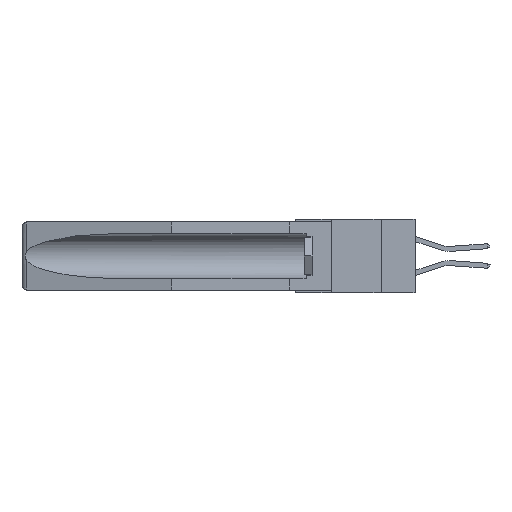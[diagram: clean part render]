
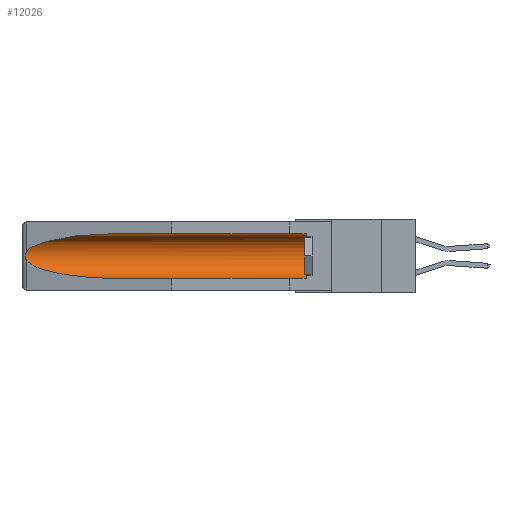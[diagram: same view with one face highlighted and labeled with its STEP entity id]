
A CAD part, left-side view. The second image highlights one B-rep face of the part: STEP entity #12026.
In plain terms, the highlighted cylindrical face has radius 2.857 mm (diameter 5.715 mm), a partial arc.
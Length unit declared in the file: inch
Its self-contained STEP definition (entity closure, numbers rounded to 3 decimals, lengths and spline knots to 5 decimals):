
#19 = CARTESIAN_POINT ( 'NONE',  ( 0.155, -0.30754, -0.059 ) ) ;
#221 = DIRECTION ( 'NONE',  ( 0., 1., 0. ) ) ;
#250 = VERTEX_POINT ( 'NONE', #28380 ) ;
#555 = EDGE_CURVE ( 'NONE', #11129, #9477, #27718, .T. ) ;
#1300 = ORIENTED_EDGE ( 'NONE', *, *, #555, .T. ) ;
#1392 = CARTESIAN_POINT ( 'NONE',  ( 0.25451, 1.48313, -0.09465 ) ) ;
#1483 = CARTESIAN_POINT ( 'NONE',  ( 0.21114, 1.30732, -0.059 ) ) ;
#3285 = DIRECTION ( 'NONE',  ( 0., 1., 0. ) ) ;
#3502 = VECTOR ( 'NONE', #3285, 39.37008 ) ;
#3849 = CARTESIAN_POINT ( 'NONE',  ( 0.155, -0.30754, -0.1715 ) ) ;
#3944 = CARTESIAN_POINT ( 'NONE',  ( 0.155, 1.07973, -0.284 ) ) ;
#4108 = CARTESIAN_POINT ( 'NONE',  ( 0.26537, 1.52718, -0.14972 ) ) ;
#4877 = VERTEX_POINT ( 'NONE', #26258 ) ;
#5162 = EDGE_CURVE ( 'NONE', #19932, #17733, #17166, .T. ) ;
#5579 = CIRCLE ( 'NONE', #13269, 0.1125 ) ;
#6385 = CARTESIAN_POINT ( 'NONE',  ( 0.26537, 1.52718, -0.19328 ) ) ;
#6817 = CARTESIAN_POINT ( 'NONE',  ( 0.155, 1.07973, -0.284 ) ) ;
#6897 =( BOUNDED_CURVE ( )  B_SPLINE_CURVE ( 3, ( #8538, #1483, #1392, #4108 ),
 .UNSPECIFIED., .F., .F. ) 
 B_SPLINE_CURVE_WITH_KNOTS ( ( 4, 4 ),
 ( 4.71239, 6.08839 ),
 .UNSPECIFIED. ) 
 CURVE ( )  GEOMETRIC_REPRESENTATION_ITEM ( )  RATIONAL_B_SPLINE_CURVE ( ( 1., 0.848, 0.848, 1. ) ) 
 REPRESENTATION_ITEM ( '' )  );
#7030 = CARTESIAN_POINT ( 'NONE',  ( 0.25451, 1.48313, -0.24835 ) ) ;
#7638 = ORIENTED_EDGE ( 'NONE', *, *, #17716, .T. ) ;
#7868 = CYLINDRICAL_SURFACE ( 'NONE', #30718, 0.1125 ) ;
#8507 = CARTESIAN_POINT ( 'NONE',  ( 0.2675, 1.53308, -0.17534 ) ) ;
#8535 = EDGE_LOOP ( 'NONE', ( #24716, #20712, #14857, #27361, #7638, #1300 ) ) ;
#8538 = CARTESIAN_POINT ( 'NONE',  ( 0.155, 1.07973, -0.059 ) ) ;
#8555 = CARTESIAN_POINT ( 'NONE',  ( 0.155, 0.126, -0.284 ) ) ;
#8702 = CARTESIAN_POINT ( 'NONE',  ( 0.2675, 1.53308, -0.16763 ) ) ;
#8983 = FACE_OUTER_BOUND ( 'NONE', #8535, .T. ) ;
#9233 = CARTESIAN_POINT ( 'NONE',  ( 0.26537, 1.52718, -0.19328 ) ) ;
#9477 = VERTEX_POINT ( 'NONE', #14952 ) ;
#11129 = VERTEX_POINT ( 'NONE', #28164 ) ;
#11135 = CARTESIAN_POINT ( 'NONE',  ( 0.155, 0.126, -0.1715 ) ) ;
#11168 = CARTESIAN_POINT ( 'NONE',  ( 0.26655, 1.53094, -0.18657 ) ) ;
#11275 = CARTESIAN_POINT ( 'NONE',  ( 0.26537, 1.52718, -0.14972 ) ) ;
#12026 = ADVANCED_FACE ( 'NONE', ( #8983 ), #7868, .F. ) ;
#13269 = AXIS2_PLACEMENT_3D ( 'NONE', #11135, #15719, #22942 ) ;
#13411 = CARTESIAN_POINT ( 'NONE',  ( 0.2673, 1.53269, -0.17917 ) ) ;
#13716 = CARTESIAN_POINT ( 'NONE',  ( 0.26654, 1.53092, -0.15636 ) ) ;
#13899 = EDGE_CURVE ( 'NONE', #9477, #250, #6897, .T. ) ;
#14857 = ORIENTED_EDGE ( 'NONE', *, *, #17355, .T. ) ;
#14886 = B_SPLINE_CURVE_WITH_KNOTS ( 'NONE', 3,
 ( #11275, #23276, #13716, #18512, #8702, #8507, #13411, #11168, #20970, #6385 ),
 .UNSPECIFIED., .F., .F.,
 ( 4, 2, 2, 2, 4 ),
 ( 0., 0.00029, 0.00058, 0.00087, 0.00117 ),
 .UNSPECIFIED. ) ;
#14952 = CARTESIAN_POINT ( 'NONE',  ( 0.155, 1.07973, -0.059 ) ) ;
#15719 = DIRECTION ( 'NONE',  ( 0., -1., 0. ) ) ;
#17166 = LINE ( 'NONE', #22568, #3502 ) ;
#17355 = EDGE_CURVE ( 'NONE', #4877, #17733, #19170, .T. ) ;
#17716 = EDGE_CURVE ( 'NONE', #19932, #11129, #5579, .T. ) ;
#17733 = VERTEX_POINT ( 'NONE', #3944 ) ;
#18512 = CARTESIAN_POINT ( 'NONE',  ( 0.2673, 1.5327, -0.16383 ) ) ;
#19170 =( BOUNDED_CURVE ( )  B_SPLINE_CURVE ( 3, ( #9233, #7030, #26312, #6817 ),
 .UNSPECIFIED., .F., .F. ) 
 B_SPLINE_CURVE_WITH_KNOTS ( ( 4, 4 ),
 ( 0.1948, 1.5708 ),
 .UNSPECIFIED. ) 
 CURVE ( )  GEOMETRIC_REPRESENTATION_ITEM ( )  RATIONAL_B_SPLINE_CURVE ( ( 1., 0.848, 0.848, 1. ) ) 
 REPRESENTATION_ITEM ( '' )  );
#19932 = VERTEX_POINT ( 'NONE', #8555 ) ;
#20712 = ORIENTED_EDGE ( 'NONE', *, *, #27794, .T. ) ;
#20970 = CARTESIAN_POINT ( 'NONE',  ( 0.26597, 1.5296, -0.19026 ) ) ;
#22568 = CARTESIAN_POINT ( 'NONE',  ( 0.155, -0.30754, -0.284 ) ) ;
#22942 = DIRECTION ( 'NONE',  ( 0., 0., 1. ) ) ;
#23276 = CARTESIAN_POINT ( 'NONE',  ( 0.26597, 1.52961, -0.15275 ) ) ;
#24716 = ORIENTED_EDGE ( 'NONE', *, *, #13899, .T. ) ;
#25446 = VECTOR ( 'NONE', #221, 39.37008 ) ;
#25679 = DIRECTION ( 'NONE',  ( 0., 1., 0. ) ) ;
#26258 = CARTESIAN_POINT ( 'NONE',  ( 0.26537, 1.52718, -0.19328 ) ) ;
#26312 = CARTESIAN_POINT ( 'NONE',  ( 0.21114, 1.30732, -0.284 ) ) ;
#27361 = ORIENTED_EDGE ( 'NONE', *, *, #5162, .F. ) ;
#27686 = DIRECTION ( 'NONE',  ( 0., 0., 1. ) ) ;
#27718 = LINE ( 'NONE', #19, #25446 ) ;
#27794 = EDGE_CURVE ( 'NONE', #250, #4877, #14886, .T. ) ;
#28164 = CARTESIAN_POINT ( 'NONE',  ( 0.155, 0.126, -0.059 ) ) ;
#28380 = CARTESIAN_POINT ( 'NONE',  ( 0.26537, 1.52718, -0.14972 ) ) ;
#30718 = AXIS2_PLACEMENT_3D ( 'NONE', #3849, #25679, #27686 ) ;
